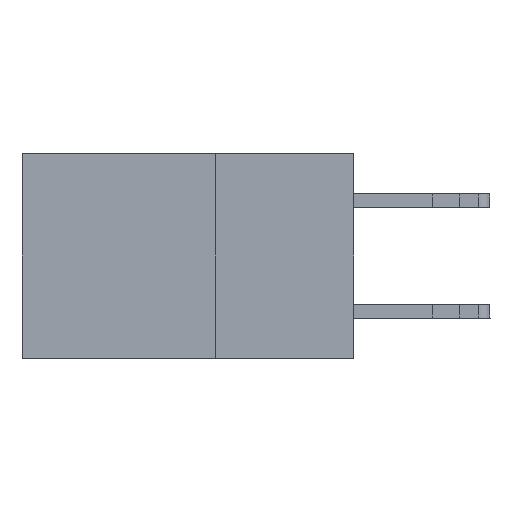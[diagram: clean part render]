
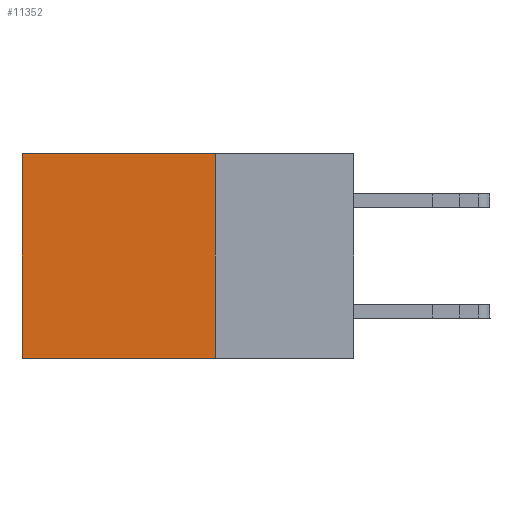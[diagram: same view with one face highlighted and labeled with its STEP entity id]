
A CAD part, left-side view. The second image highlights one B-rep face of the part: STEP entity #11352.
In plain terms, the highlighted planar face has unit normal (-1, 0, 0).
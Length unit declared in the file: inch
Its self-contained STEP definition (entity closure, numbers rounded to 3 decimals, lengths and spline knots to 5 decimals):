
#27 = LINE ( 'NONE', #4808, #13801 ) ;
#72 = ORIENTED_EDGE ( 'NONE', *, *, #13368, .F. ) ;
#126 = PLANE ( 'NONE',  #11468 ) ;
#375 = ORIENTED_EDGE ( 'NONE', *, *, #1598, .T. ) ;
#734 = CARTESIAN_POINT ( 'NONE',  ( 0.2875, 0.25, 0. ) ) ;
#1215 = VERTEX_POINT ( 'NONE', #734 ) ;
#1294 = DIRECTION ( 'NONE',  ( 0., 0., -1. ) ) ;
#1298 = CARTESIAN_POINT ( 'NONE',  ( 0.2875, 0.25, 0. ) ) ;
#1340 = EDGE_CURVE ( 'NONE', #1215, #10537, #3625, .T. ) ;
#1466 = VECTOR ( 'NONE', #5848, 39.37008 ) ;
#1468 = DIRECTION ( 'NONE',  ( 0., 0., -1. ) ) ;
#1598 = EDGE_CURVE ( 'NONE', #10537, #4386, #15901, .T. ) ;
#2002 = VECTOR ( 'NONE', #14459, 39.37008 ) ;
#2279 = CARTESIAN_POINT ( 'NONE',  ( 0.2875, 0.6, 0. ) ) ;
#3625 = LINE ( 'NONE', #5115, #9449 ) ;
#3744 = ORIENTED_EDGE ( 'NONE', *, *, #9334, .F. ) ;
#4323 = ORIENTED_EDGE ( 'NONE', *, *, #1340, .T. ) ;
#4386 = VERTEX_POINT ( 'NONE', #10809 ) ;
#4808 = CARTESIAN_POINT ( 'NONE',  ( 0.2875, 0.25, 0. ) ) ;
#5115 = CARTESIAN_POINT ( 'NONE',  ( 0.2875, 0.25, 0. ) ) ;
#5204 = DIRECTION ( 'NONE',  ( 0., 1., 0. ) ) ;
#5848 = DIRECTION ( 'NONE',  ( 0., 0., -1. ) ) ;
#6198 = VERTEX_POINT ( 'NONE', #9391 ) ;
#6970 = LINE ( 'NONE', #10733, #2002 ) ;
#9030 = FACE_OUTER_BOUND ( 'NONE', #13498, .T. ) ;
#9334 = EDGE_CURVE ( 'NONE', #6198, #4386, #6970, .T. ) ;
#9391 = CARTESIAN_POINT ( 'NONE',  ( 0.2875, 0.25, -0.37 ) ) ;
#9449 = VECTOR ( 'NONE', #5204, 39.37008 ) ;
#10537 = VERTEX_POINT ( 'NONE', #10580 ) ;
#10580 = CARTESIAN_POINT ( 'NONE',  ( 0.2875, 0.6, 0. ) ) ;
#10733 = CARTESIAN_POINT ( 'NONE',  ( 0.2875, 0.25, -0.37 ) ) ;
#10809 = CARTESIAN_POINT ( 'NONE',  ( 0.2875, 0.6, -0.37 ) ) ;
#11352 = ADVANCED_FACE ( 'NONE', ( #9030 ), #126, .F. ) ;
#11468 = AXIS2_PLACEMENT_3D ( 'NONE', #1298, #11614, #1468 ) ;
#11614 = DIRECTION ( 'NONE',  ( 1., 0., 0. ) ) ;
#13368 = EDGE_CURVE ( 'NONE', #1215, #6198, #27, .T. ) ;
#13498 = EDGE_LOOP ( 'NONE', ( #375, #3744, #72, #4323 ) ) ;
#13801 = VECTOR ( 'NONE', #1294, 39.37008 ) ;
#14459 = DIRECTION ( 'NONE',  ( 0., 1., 0. ) ) ;
#15901 = LINE ( 'NONE', #2279, #1466 ) ;
